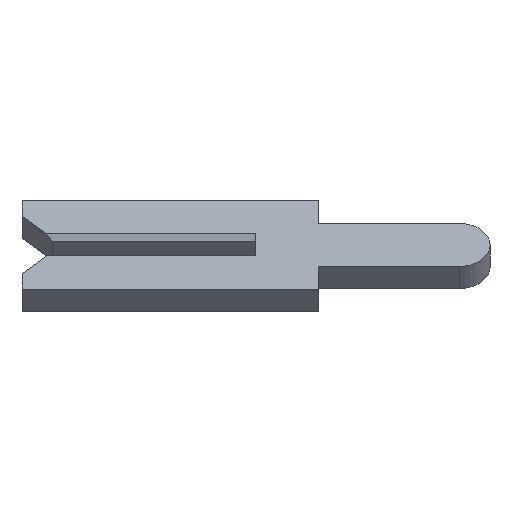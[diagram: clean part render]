
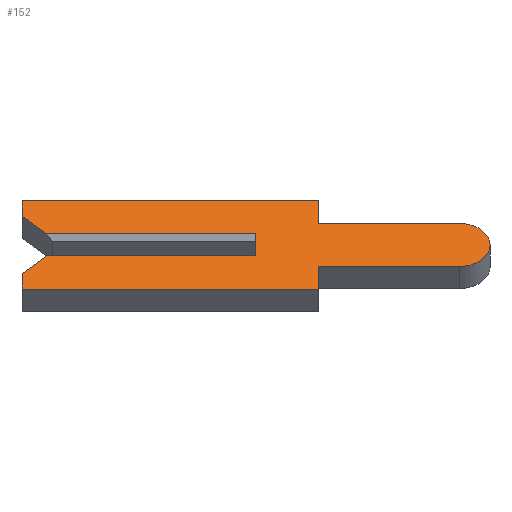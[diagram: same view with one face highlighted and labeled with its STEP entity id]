
A CAD part, left-side view. The second image highlights one B-rep face of the part: STEP entity #152.
In plain terms, the highlighted face is planar.
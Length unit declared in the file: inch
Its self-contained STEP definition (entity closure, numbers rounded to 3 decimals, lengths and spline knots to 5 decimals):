
#4 = VERTEX_POINT ( 'NONE', #726 ) ;
#5 = EDGE_CURVE ( 'NONE', #459, #497, #233, .T. ) ;
#11 = PLANE ( 'NONE',  #89 ) ;
#37 = ORIENTED_EDGE ( 'NONE', *, *, #5, .F. ) ;
#53 = EDGE_CURVE ( 'NONE', #236, #4, #255, .T. ) ;
#58 = VECTOR ( 'NONE', #529, 39.37008 ) ;
#70 = VECTOR ( 'NONE', #95, 39.37008 ) ;
#80 = VECTOR ( 'NONE', #411, 39.37008 ) ;
#89 = AXIS2_PLACEMENT_3D ( 'NONE', #303, #795, #363 ) ;
#92 = CIRCLE ( 'NONE', #188, 0.0195 ) ;
#95 = DIRECTION ( 'NONE',  ( 0., -0.707, 0.707 ) ) ;
#99 = EDGE_CURVE ( 'NONE', #474, #261, #418, .T. ) ;
#100 = VERTEX_POINT ( 'NONE', #737 ) ;
#105 = DIRECTION ( 'NONE',  ( 0., 1., 0. ) ) ;
#106 = EDGE_CURVE ( 'NONE', #497, #429, #194, .T. ) ;
#107 = CARTESIAN_POINT ( 'NONE',  ( -0.01, 0.15, 0.026 ) ) ;
#109 = CARTESIAN_POINT ( 'NONE',  ( -0.01, 0.15, 0.04 ) ) ;
#110 = ORIENTED_EDGE ( 'NONE', *, *, #668, .F. ) ;
#115 = DIRECTION ( 'NONE',  ( 0., 1., 0. ) ) ;
#119 = LINE ( 'NONE', #137, #495 ) ;
#133 = EDGE_CURVE ( 'NONE', #429, #100, #506, .T. ) ;
#136 = VERTEX_POINT ( 'NONE', #872 ) ;
#137 = CARTESIAN_POINT ( 'NONE',  ( -0.01, 0., 0.0065 ) ) ;
#145 = EDGE_CURVE ( 'NONE', #4, #528, #257, .T. ) ;
#152 = ADVANCED_FACE ( 'NONE', ( #272 ), #11, .F. ) ;
#168 = ORIENTED_EDGE ( 'NONE', *, *, #53, .F. ) ;
#173 = CARTESIAN_POINT ( 'NONE',  ( -0.01, -0.1305, -0.0195 ) ) ;
#175 = CARTESIAN_POINT ( 'NONE',  ( -0.01, -0.04, 0.04 ) ) ;
#179 = LINE ( 'NONE', #521, #185 ) ;
#184 = CARTESIAN_POINT ( 'NONE',  ( -0.01, 0., -0.01 ) ) ;
#185 = VECTOR ( 'NONE', #105, 39.37008 ) ;
#187 = CARTESIAN_POINT ( 'NONE',  ( -0.01, -0.1305, 0.0195 ) ) ;
#188 = AXIS2_PLACEMENT_3D ( 'NONE', #812, #520, #743 ) ;
#192 = CARTESIAN_POINT ( 'NONE',  ( -0.01, -0.04, -0.04 ) ) ;
#194 = LINE ( 'NONE', #670, #58 ) ;
#197 = CARTESIAN_POINT ( 'NONE',  ( -0.01, 0.1305, 0.0065 ) ) ;
#209 = ORIENTED_EDGE ( 'NONE', *, *, #828, .F. ) ;
#223 = ORIENTED_EDGE ( 'NONE', *, *, #382, .F. ) ;
#233 = LINE ( 'NONE', #250, #585 ) ;
#236 = VERTEX_POINT ( 'NONE', #728 ) ;
#240 = LINE ( 'NONE', #192, #472 ) ;
#250 = CARTESIAN_POINT ( 'NONE',  ( -0.01, 0.15, 0.026 ) ) ;
#255 = LINE ( 'NONE', #317, #70 ) ;
#257 = LINE ( 'NONE', #647, #732 ) ;
#258 = DIRECTION ( 'NONE',  ( 0., 0., -1. ) ) ;
#261 = VERTEX_POINT ( 'NONE', #545 ) ;
#272 = FACE_OUTER_BOUND ( 'NONE', #765, .T. ) ;
#291 = ORIENTED_EDGE ( 'NONE', *, *, #133, .F. ) ;
#297 = ORIENTED_EDGE ( 'NONE', *, *, #822, .F. ) ;
#303 = CARTESIAN_POINT ( 'NONE',  ( -0.01, -0.1305, 0. ) ) ;
#317 = CARTESIAN_POINT ( 'NONE',  ( -0.01, 0.1305, -0.0065 ) ) ;
#322 = DIRECTION ( 'NONE',  ( 0., 0., 1. ) ) ;
#323 = CARTESIAN_POINT ( 'NONE',  ( -0.01, 0.134, 0.01 ) ) ;
#324 = ORIENTED_EDGE ( 'NONE', *, *, #145, .F. ) ;
#328 = CARTESIAN_POINT ( 'NONE',  ( -0.01, -0.04, -0.0195 ) ) ;
#331 = VECTOR ( 'NONE', #635, 39.37008 ) ;
#342 = CARTESIAN_POINT ( 'NONE',  ( -0.01, 0.15, -0.026 ) ) ;
#354 = VERTEX_POINT ( 'NONE', #173 ) ;
#363 = DIRECTION ( 'NONE',  ( 0., 0., -1. ) ) ;
#382 = EDGE_CURVE ( 'NONE', #354, #505, #179, .T. ) ;
#397 = EDGE_CURVE ( 'NONE', #603, #354, #92, .T. ) ;
#401 = DIRECTION ( 'NONE',  ( 0., -1., 0. ) ) ;
#403 = VECTOR ( 'NONE', #115, 39.37008 ) ;
#406 = VECTOR ( 'NONE', #258, 39.37008 ) ;
#411 = DIRECTION ( 'NONE',  ( 0., 0., 1. ) ) ;
#418 = LINE ( 'NONE', #452, #565 ) ;
#429 = VERTEX_POINT ( 'NONE', #175 ) ;
#433 = DIRECTION ( 'NONE',  ( 0., -1., 0. ) ) ;
#450 = LINE ( 'NONE', #342, #80 ) ;
#452 = CARTESIAN_POINT ( 'NONE',  ( -0.01, 0.15, 0.01 ) ) ;
#459 = VERTEX_POINT ( 'NONE', #107 ) ;
#472 = VECTOR ( 'NONE', #687, 39.37008 ) ;
#474 = VERTEX_POINT ( 'NONE', #323 ) ;
#482 = CARTESIAN_POINT ( 'NONE',  ( -0.01, -0.04, 0.0195 ) ) ;
#495 = VECTOR ( 'NONE', #697, 39.37008 ) ;
#497 = VERTEX_POINT ( 'NONE', #109 ) ;
#505 = VERTEX_POINT ( 'NONE', #328 ) ;
#506 = LINE ( 'NONE', #678, #406 ) ;
#520 = DIRECTION ( 'NONE',  ( 1., 0., 0. ) ) ;
#521 = CARTESIAN_POINT ( 'NONE',  ( -0.01, -0.04, -0.0195 ) ) ;
#528 = VERTEX_POINT ( 'NONE', #184 ) ;
#529 = DIRECTION ( 'NONE',  ( 0., -1., 0. ) ) ;
#542 = ORIENTED_EDGE ( 'NONE', *, *, #682, .F. ) ;
#545 = CARTESIAN_POINT ( 'NONE',  ( -0.01, 0., 0.01 ) ) ;
#565 = VECTOR ( 'NONE', #401, 39.37008 ) ;
#568 = VERTEX_POINT ( 'NONE', #882 ) ;
#585 = VECTOR ( 'NONE', #322, 39.37008 ) ;
#590 = EDGE_CURVE ( 'NONE', #136, #568, #659, .T. ) ;
#603 = VERTEX_POINT ( 'NONE', #187 ) ;
#635 = DIRECTION ( 'NONE',  ( 0., -1., 0. ) ) ;
#637 = LINE ( 'NONE', #197, #766 ) ;
#647 = CARTESIAN_POINT ( 'NONE',  ( -0.01, -0.1305, -0.01 ) ) ;
#649 = ORIENTED_EDGE ( 'NONE', *, *, #397, .F. ) ;
#659 = LINE ( 'NONE', #679, #403 ) ;
#668 = EDGE_CURVE ( 'NONE', #505, #136, #240, .T. ) ;
#670 = CARTESIAN_POINT ( 'NONE',  ( -0.01, 0.15, 0.04 ) ) ;
#678 = CARTESIAN_POINT ( 'NONE',  ( -0.01, -0.04, 0.04 ) ) ;
#679 = CARTESIAN_POINT ( 'NONE',  ( -0.01, 0.15, -0.04 ) ) ;
#682 = EDGE_CURVE ( 'NONE', #100, #603, #840, .T. ) ;
#687 = DIRECTION ( 'NONE',  ( 0., 0., -1. ) ) ;
#697 = DIRECTION ( 'NONE',  ( 0., 0., 1. ) ) ;
#709 = ORIENTED_EDGE ( 'NONE', *, *, #590, .F. ) ;
#720 = ORIENTED_EDGE ( 'NONE', *, *, #99, .T. ) ;
#726 = CARTESIAN_POINT ( 'NONE',  ( -0.01, 0.134, -0.01 ) ) ;
#728 = CARTESIAN_POINT ( 'NONE',  ( -0.01, 0.15, -0.026 ) ) ;
#732 = VECTOR ( 'NONE', #433, 39.37008 ) ;
#737 = CARTESIAN_POINT ( 'NONE',  ( -0.01, -0.04, 0.0195 ) ) ;
#743 = DIRECTION ( 'NONE',  ( 0., 0., -1. ) ) ;
#765 = EDGE_LOOP ( 'NONE', ( #720, #209, #324, #168, #297, #709, #110, #223, #649, #542, #291, #829, #37, #816 ) ) ;
#766 = VECTOR ( 'NONE', #772, 39.37008 ) ;
#772 = DIRECTION ( 'NONE',  ( 0., 0.707, 0.707 ) ) ;
#795 = DIRECTION ( 'NONE',  ( 1., 0., 0. ) ) ;
#797 = EDGE_CURVE ( 'NONE', #474, #459, #637, .T. ) ;
#812 = CARTESIAN_POINT ( 'NONE',  ( -0.01, -0.1305, 0. ) ) ;
#816 = ORIENTED_EDGE ( 'NONE', *, *, #797, .F. ) ;
#822 = EDGE_CURVE ( 'NONE', #568, #236, #450, .T. ) ;
#828 = EDGE_CURVE ( 'NONE', #528, #261, #119, .T. ) ;
#829 = ORIENTED_EDGE ( 'NONE', *, *, #106, .F. ) ;
#840 = LINE ( 'NONE', #482, #331 ) ;
#872 = CARTESIAN_POINT ( 'NONE',  ( -0.01, -0.04, -0.04 ) ) ;
#882 = CARTESIAN_POINT ( 'NONE',  ( -0.01, 0.15, -0.04 ) ) ;
